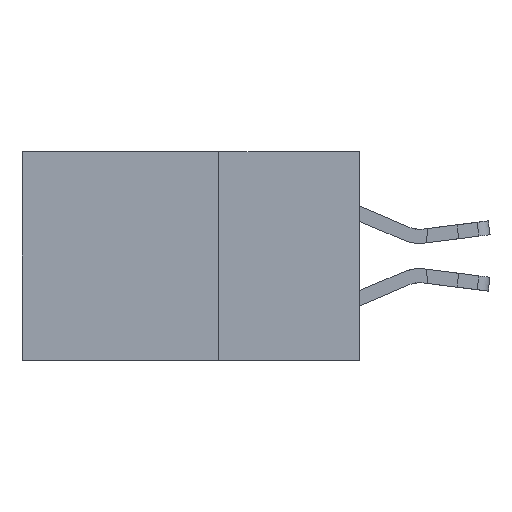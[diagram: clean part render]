
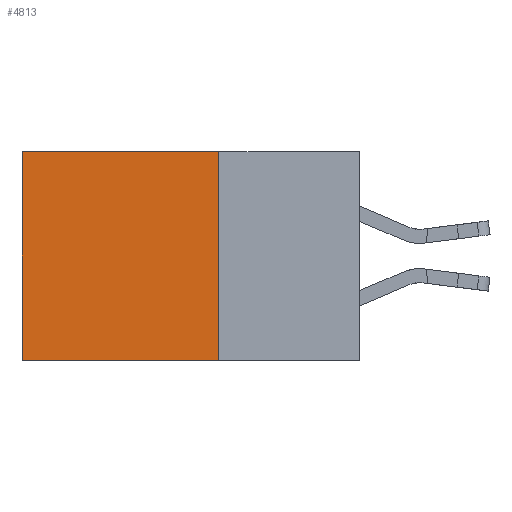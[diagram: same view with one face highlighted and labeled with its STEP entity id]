
A CAD part, left-side view. The second image highlights one B-rep face of the part: STEP entity #4813.
In plain terms, the highlighted planar face has unit normal (-1, 0, 0).
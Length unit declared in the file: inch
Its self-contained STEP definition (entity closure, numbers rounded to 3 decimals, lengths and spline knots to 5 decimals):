
#174 = FACE_OUTER_BOUND ( 'NONE', #8512, .T. ) ;
#1059 = VECTOR ( 'NONE', #8553, 39.37008 ) ;
#1202 = LINE ( 'NONE', #11679, #7537 ) ;
#1499 = DIRECTION ( 'NONE',  ( 0., 0., -1. ) ) ;
#2183 = VERTEX_POINT ( 'NONE', #3419 ) ;
#3096 = LINE ( 'NONE', #9956, #13524 ) ;
#3345 = AXIS2_PLACEMENT_3D ( 'NONE', #15948, #9486, #1499 ) ;
#3405 = DIRECTION ( 'NONE',  ( 0., 1., 0. ) ) ;
#3419 = CARTESIAN_POINT ( 'NONE',  ( 0.2875, 0.25, 0. ) ) ;
#4813 = ADVANCED_FACE ( 'NONE', ( #174 ), #8185, .F. ) ;
#5852 = EDGE_CURVE ( 'NONE', #7387, #13107, #12763, .T. ) ;
#7387 = VERTEX_POINT ( 'NONE', #14596 ) ;
#7537 = VECTOR ( 'NONE', #12981, 39.37008 ) ;
#7560 = EDGE_CURVE ( 'NONE', #2183, #10487, #3096, .T. ) ;
#8185 = PLANE ( 'NONE',  #3345 ) ;
#8512 = EDGE_LOOP ( 'NONE', ( #11565, #9409, #14435, #9843 ) ) ;
#8553 = DIRECTION ( 'NONE',  ( 0., 0., -1. ) ) ;
#9350 = VECTOR ( 'NONE', #11911, 39.37008 ) ;
#9409 = ORIENTED_EDGE ( 'NONE', *, *, #5852, .F. ) ;
#9486 = DIRECTION ( 'NONE',  ( 1., 0., 0. ) ) ;
#9796 = CARTESIAN_POINT ( 'NONE',  ( 0.2875, 0.6, 0. ) ) ;
#9843 = ORIENTED_EDGE ( 'NONE', *, *, #7560, .T. ) ;
#9956 = CARTESIAN_POINT ( 'NONE',  ( 0.2875, 0.25, 0. ) ) ;
#10487 = VERTEX_POINT ( 'NONE', #10983 ) ;
#10983 = CARTESIAN_POINT ( 'NONE',  ( 0.2875, 0.6, 0. ) ) ;
#11164 = EDGE_CURVE ( 'NONE', #2183, #7387, #1202, .T. ) ;
#11565 = ORIENTED_EDGE ( 'NONE', *, *, #15354, .T. ) ;
#11679 = CARTESIAN_POINT ( 'NONE',  ( 0.2875, 0.25, 0. ) ) ;
#11911 = DIRECTION ( 'NONE',  ( 0., 1., 0. ) ) ;
#12010 = LINE ( 'NONE', #9796, #1059 ) ;
#12763 = LINE ( 'NONE', #15805, #9350 ) ;
#12981 = DIRECTION ( 'NONE',  ( 0., 0., -1. ) ) ;
#12986 = CARTESIAN_POINT ( 'NONE',  ( 0.2875, 0.6, -0.37 ) ) ;
#13107 = VERTEX_POINT ( 'NONE', #12986 ) ;
#13524 = VECTOR ( 'NONE', #3405, 39.37008 ) ;
#14435 = ORIENTED_EDGE ( 'NONE', *, *, #11164, .F. ) ;
#14596 = CARTESIAN_POINT ( 'NONE',  ( 0.2875, 0.25, -0.37 ) ) ;
#15354 = EDGE_CURVE ( 'NONE', #10487, #13107, #12010, .T. ) ;
#15805 = CARTESIAN_POINT ( 'NONE',  ( 0.2875, 0.25, -0.37 ) ) ;
#15948 = CARTESIAN_POINT ( 'NONE',  ( 0.2875, 0.25, 0. ) ) ;
